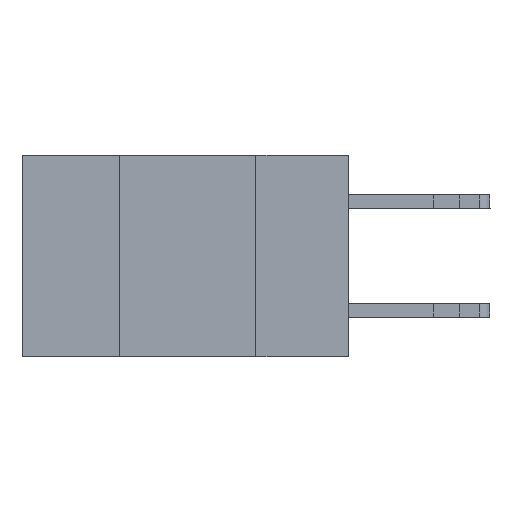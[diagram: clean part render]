
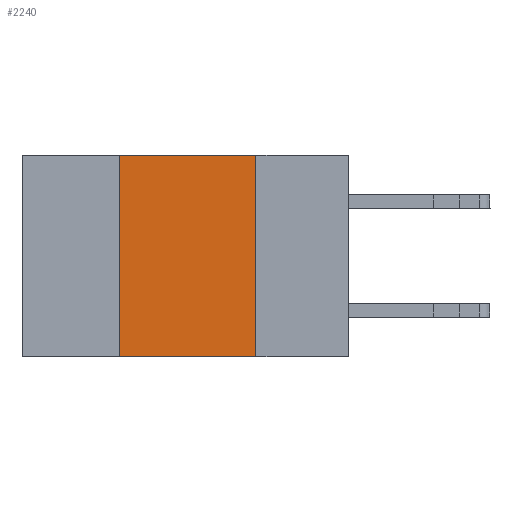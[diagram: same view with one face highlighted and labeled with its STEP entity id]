
A CAD part, left-side view. The second image highlights one B-rep face of the part: STEP entity #2240.
In plain terms, the highlighted planar face has unit normal (-1, 0, 0).
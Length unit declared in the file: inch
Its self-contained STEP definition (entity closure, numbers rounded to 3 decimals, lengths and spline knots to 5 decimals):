
#9 = EDGE_CURVE ( 'NONE', #4259, #2643, #9379, .T. ) ;
#26 = LINE ( 'NONE', #9382, #8180 ) ;
#199 = VERTEX_POINT ( 'NONE', #295 ) ;
#295 = CARTESIAN_POINT ( 'NONE',  ( 0., 0.42, 0. ) ) ;
#443 = VERTEX_POINT ( 'NONE', #6300 ) ;
#479 = ORIENTED_EDGE ( 'NONE', *, *, #10049, .F. ) ;
#1570 = PLANE ( 'NONE',  #10178 ) ;
#1764 = ORIENTED_EDGE ( 'NONE', *, *, #4587, .F. ) ;
#1807 = CARTESIAN_POINT ( 'NONE',  ( 0., 0.6, 0. ) ) ;
#2031 = VECTOR ( 'NONE', #4703, 39.37008 ) ;
#2115 = CARTESIAN_POINT ( 'NONE',  ( 0., 0.17, -0.37 ) ) ;
#2240 = ADVANCED_FACE ( 'NONE', ( #10225 ), #1570, .F. ) ;
#2643 = VERTEX_POINT ( 'NONE', #4251 ) ;
#3837 = DIRECTION ( 'NONE',  ( 0., -1., 0. ) ) ;
#3983 = EDGE_LOOP ( 'NONE', ( #4961, #1764, #479, #10158 ) ) ;
#4251 = CARTESIAN_POINT ( 'NONE',  ( 0., 0.17, -0.37 ) ) ;
#4259 = VERTEX_POINT ( 'NONE', #4307 ) ;
#4307 = CARTESIAN_POINT ( 'NONE',  ( 0., 0.17, 0. ) ) ;
#4587 = EDGE_CURVE ( 'NONE', #199, #4259, #6321, .T. ) ;
#4703 = DIRECTION ( 'NONE',  ( 0., 0., -1. ) ) ;
#4961 = ORIENTED_EDGE ( 'NONE', *, *, #9, .F. ) ;
#5301 = VECTOR ( 'NONE', #8181, 39.37008 ) ;
#5973 = VECTOR ( 'NONE', #9355, 39.37008 ) ;
#6300 = CARTESIAN_POINT ( 'NONE',  ( 0., 0.42, -0.37 ) ) ;
#6321 = LINE ( 'NONE', #11077, #5301 ) ;
#6676 = LINE ( 'NONE', #10443, #5973 ) ;
#7426 = DIRECTION ( 'NONE',  ( 1., 0., 0. ) ) ;
#8180 = VECTOR ( 'NONE', #3837, 39.37008 ) ;
#8181 = DIRECTION ( 'NONE',  ( 0., -1., 0. ) ) ;
#9040 = DIRECTION ( 'NONE',  ( 0., 0., -1. ) ) ;
#9355 = DIRECTION ( 'NONE',  ( 0., 0., 1. ) ) ;
#9379 = LINE ( 'NONE', #2115, #2031 ) ;
#9382 = CARTESIAN_POINT ( 'NONE',  ( 0., 0.6, -0.37 ) ) ;
#10049 = EDGE_CURVE ( 'NONE', #443, #199, #6676, .T. ) ;
#10158 = ORIENTED_EDGE ( 'NONE', *, *, #12161, .T. ) ;
#10178 = AXIS2_PLACEMENT_3D ( 'NONE', #1807, #7426, #9040 ) ;
#10225 = FACE_OUTER_BOUND ( 'NONE', #3983, .T. ) ;
#10443 = CARTESIAN_POINT ( 'NONE',  ( 0., 0.42, -0.37 ) ) ;
#11077 = CARTESIAN_POINT ( 'NONE',  ( 0., 0.6, 0. ) ) ;
#12161 = EDGE_CURVE ( 'NONE', #443, #2643, #26, .T. ) ;
